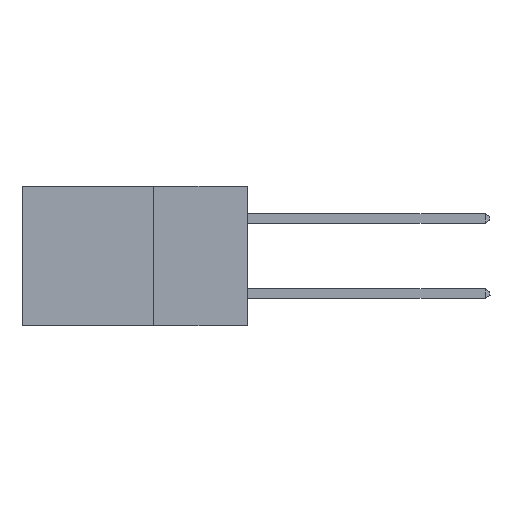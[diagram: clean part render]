
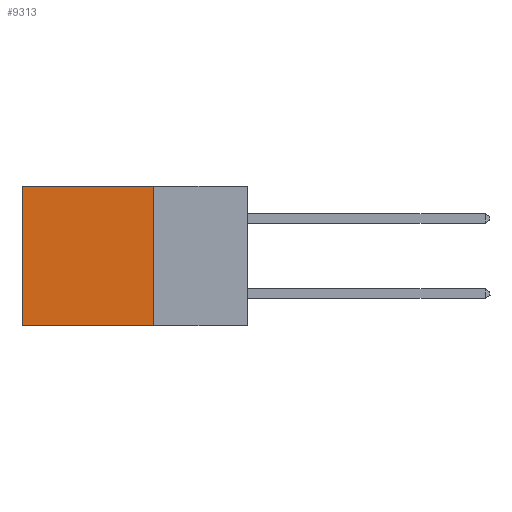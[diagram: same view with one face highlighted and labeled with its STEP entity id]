
A CAD part, left-side view. The second image highlights one B-rep face of the part: STEP entity #9313.
In plain terms, the highlighted planar face has unit normal (-1, 0, 0).
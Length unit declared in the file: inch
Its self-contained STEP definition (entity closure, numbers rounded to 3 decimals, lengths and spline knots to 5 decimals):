
#699 = DIRECTION ( 'NONE',  ( 0., 1., 0. ) ) ;
#768 = DIRECTION ( 'NONE',  ( 0., 0., -1. ) ) ;
#835 = CARTESIAN_POINT ( 'NONE',  ( 0.298, 0.6, 0. ) ) ;
#928 = CARTESIAN_POINT ( 'NONE',  ( 0.298, 0.25, 0. ) ) ;
#989 = PLANE ( 'NONE',  #3676 ) ;
#1170 = ORIENTED_EDGE ( 'NONE', *, *, #15285, .T. ) ;
#1420 = LINE ( 'NONE', #14522, #13131 ) ;
#1548 = FACE_OUTER_BOUND ( 'NONE', #7173, .T. ) ;
#1916 = ORIENTED_EDGE ( 'NONE', *, *, #5836, .F. ) ;
#2856 = EDGE_CURVE ( 'NONE', #6921, #8602, #1420, .T. ) ;
#3676 = AXIS2_PLACEMENT_3D ( 'NONE', #928, #16540, #16364 ) ;
#3777 = LINE ( 'NONE', #6898, #13072 ) ;
#4707 = VERTEX_POINT ( 'NONE', #6173 ) ;
#4754 = VECTOR ( 'NONE', #8539, 39.37008 ) ;
#5388 = CARTESIAN_POINT ( 'NONE',  ( 0.298, 0.6, -0.37 ) ) ;
#5836 = EDGE_CURVE ( 'NONE', #6921, #4707, #19439, .T. ) ;
#6173 = CARTESIAN_POINT ( 'NONE',  ( 0.298, 0.25, -0.37 ) ) ;
#6465 = ORIENTED_EDGE ( 'NONE', *, *, #2856, .T. ) ;
#6898 = CARTESIAN_POINT ( 'NONE',  ( 0.298, 0.6, 0. ) ) ;
#6921 = VERTEX_POINT ( 'NONE', #8043 ) ;
#7173 = EDGE_LOOP ( 'NONE', ( #1170, #13133, #1916, #6465 ) ) ;
#8043 = CARTESIAN_POINT ( 'NONE',  ( 0.298, 0.25, 0. ) ) ;
#8539 = DIRECTION ( 'NONE',  ( 0., 1., 0. ) ) ;
#8565 = VERTEX_POINT ( 'NONE', #5388 ) ;
#8602 = VERTEX_POINT ( 'NONE', #835 ) ;
#8702 = VECTOR ( 'NONE', #12277, 39.37008 ) ;
#9313 = ADVANCED_FACE ( 'NONE', ( #1548 ), #989, .F. ) ;
#12277 = DIRECTION ( 'NONE',  ( 0., 0., -1. ) ) ;
#12360 = CARTESIAN_POINT ( 'NONE',  ( 0.298, 0.25, 0. ) ) ;
#13072 = VECTOR ( 'NONE', #768, 39.37008 ) ;
#13131 = VECTOR ( 'NONE', #699, 39.37008 ) ;
#13133 = ORIENTED_EDGE ( 'NONE', *, *, #14449, .F. ) ;
#14058 = LINE ( 'NONE', #17921, #4754 ) ;
#14449 = EDGE_CURVE ( 'NONE', #4707, #8565, #14058, .T. ) ;
#14522 = CARTESIAN_POINT ( 'NONE',  ( 0.298, 0.25, 0. ) ) ;
#15285 = EDGE_CURVE ( 'NONE', #8602, #8565, #3777, .T. ) ;
#16364 = DIRECTION ( 'NONE',  ( 0., 0., -1. ) ) ;
#16540 = DIRECTION ( 'NONE',  ( 1., 0., 0. ) ) ;
#17921 = CARTESIAN_POINT ( 'NONE',  ( 0.298, 0.25, -0.37 ) ) ;
#19439 = LINE ( 'NONE', #12360, #8702 ) ;
